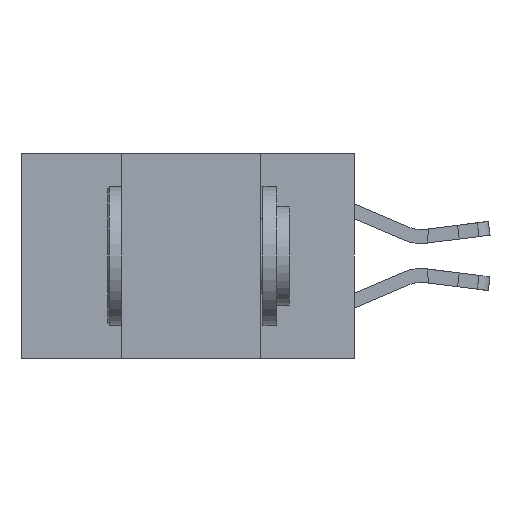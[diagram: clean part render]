
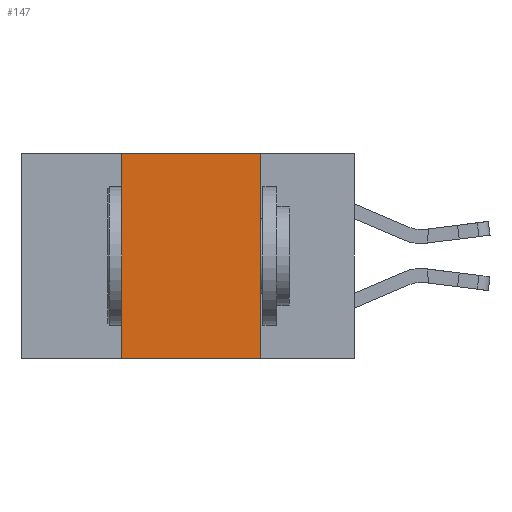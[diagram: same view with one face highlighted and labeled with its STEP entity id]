
A CAD part, left-side view. The second image highlights one B-rep face of the part: STEP entity #147.
In plain terms, the highlighted planar face has unit normal (-1, 0, 0).
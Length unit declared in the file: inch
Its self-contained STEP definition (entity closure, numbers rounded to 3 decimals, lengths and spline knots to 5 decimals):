
#60 = VERTEX_POINT ( 'NONE', #4982 ) ;
#147 = ADVANCED_FACE ( 'NONE', ( #4242 ), #1361, .F. ) ;
#469 = ORIENTED_EDGE ( 'NONE', *, *, #6585, .F. ) ;
#487 = CARTESIAN_POINT ( 'NONE',  ( 0., 0.42, 0. ) ) ;
#1361 = PLANE ( 'NONE',  #5798 ) ;
#1371 = DIRECTION ( 'NONE',  ( 0., -1., 0. ) ) ;
#1471 = EDGE_LOOP ( 'NONE', ( #7446, #8016, #469, #2528 ) ) ;
#1623 = CARTESIAN_POINT ( 'NONE',  ( 0., 0.42, -0.37 ) ) ;
#1846 = CARTESIAN_POINT ( 'NONE',  ( 0., 0.17, 0. ) ) ;
#2424 = CARTESIAN_POINT ( 'NONE',  ( 0., 0.6, 0. ) ) ;
#2528 = ORIENTED_EDGE ( 'NONE', *, *, #5929, .T. ) ;
#2539 = EDGE_CURVE ( 'NONE', #5808, #3772, #5317, .T. ) ;
#3373 = LINE ( 'NONE', #1623, #9295 ) ;
#3772 = VERTEX_POINT ( 'NONE', #3812 ) ;
#3812 = CARTESIAN_POINT ( 'NONE',  ( 0., 0.17, -0.37 ) ) ;
#4205 = CARTESIAN_POINT ( 'NONE',  ( 0., 0.6, -0.37 ) ) ;
#4242 = FACE_OUTER_BOUND ( 'NONE', #1471, .T. ) ;
#4982 = CARTESIAN_POINT ( 'NONE',  ( 0., 0.42, -0.37 ) ) ;
#5317 = LINE ( 'NONE', #6451, #11191 ) ;
#5798 = AXIS2_PLACEMENT_3D ( 'NONE', #2424, #8009, #8066 ) ;
#5808 = VERTEX_POINT ( 'NONE', #1846 ) ;
#5929 = EDGE_CURVE ( 'NONE', #60, #3772, #10793, .T. ) ;
#6384 = DIRECTION ( 'NONE',  ( 0., 0., -1. ) ) ;
#6451 = CARTESIAN_POINT ( 'NONE',  ( 0., 0.17, -0.37 ) ) ;
#6549 = EDGE_CURVE ( 'NONE', #6994, #5808, #8018, .T. ) ;
#6585 = EDGE_CURVE ( 'NONE', #60, #6994, #3373, .T. ) ;
#6994 = VERTEX_POINT ( 'NONE', #487 ) ;
#7146 = DIRECTION ( 'NONE',  ( 0., 0., 1. ) ) ;
#7446 = ORIENTED_EDGE ( 'NONE', *, *, #2539, .F. ) ;
#8009 = DIRECTION ( 'NONE',  ( 1., 0., 0. ) ) ;
#8016 = ORIENTED_EDGE ( 'NONE', *, *, #6549, .F. ) ;
#8018 = LINE ( 'NONE', #11821, #11833 ) ;
#8066 = DIRECTION ( 'NONE',  ( 0., 0., -1. ) ) ;
#9295 = VECTOR ( 'NONE', #7146, 39.37008 ) ;
#10793 = LINE ( 'NONE', #4205, #11428 ) ;
#11191 = VECTOR ( 'NONE', #6384, 39.37008 ) ;
#11428 = VECTOR ( 'NONE', #11717, 39.37008 ) ;
#11717 = DIRECTION ( 'NONE',  ( 0., -1., 0. ) ) ;
#11821 = CARTESIAN_POINT ( 'NONE',  ( 0., 0.6, 0. ) ) ;
#11833 = VECTOR ( 'NONE', #1371, 39.37008 ) ;
